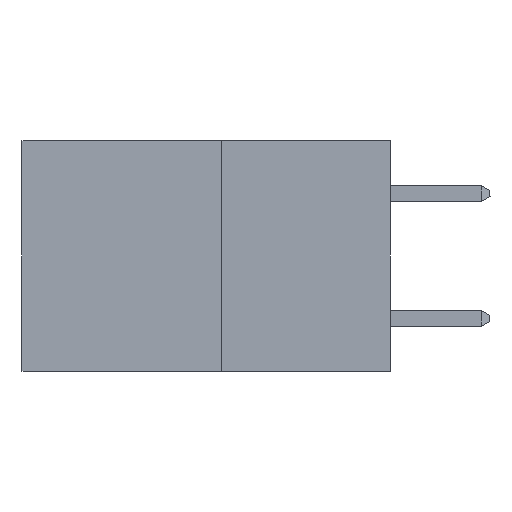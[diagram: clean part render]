
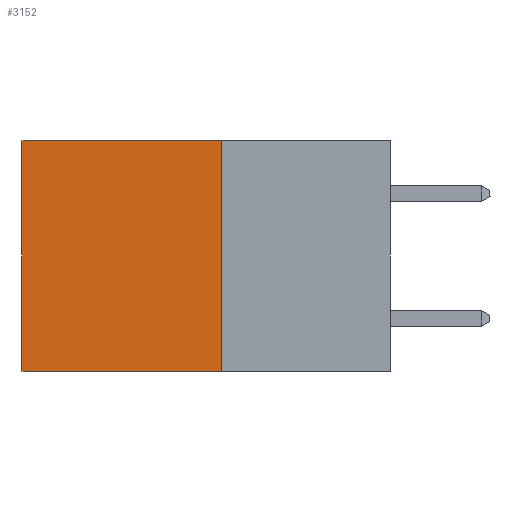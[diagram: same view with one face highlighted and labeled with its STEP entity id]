
A CAD part, left-side view. The second image highlights one B-rep face of the part: STEP entity #3152.
In plain terms, the highlighted planar face has unit normal (-1, 0, 0).
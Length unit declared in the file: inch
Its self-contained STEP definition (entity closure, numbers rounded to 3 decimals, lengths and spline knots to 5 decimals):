
#221 = LINE ( 'NONE', #6508, #7638 ) ;
#375 = DIRECTION ( 'NONE',  ( 0., 1., 0. ) ) ;
#657 = LINE ( 'NONE', #3395, #8274 ) ;
#1483 = AXIS2_PLACEMENT_3D ( 'NONE', #6103, #1688, #1674 ) ;
#1544 = LINE ( 'NONE', #1906, #3547 ) ;
#1674 = DIRECTION ( 'NONE',  ( 0., 0., -1. ) ) ;
#1688 = DIRECTION ( 'NONE',  ( 1., 0., 0. ) ) ;
#1906 = CARTESIAN_POINT ( 'NONE',  ( 0.277, 0.27, 0. ) ) ;
#1997 = ORIENTED_EDGE ( 'NONE', *, *, #3119, .F. ) ;
#2103 = VERTEX_POINT ( 'NONE', #8657 ) ;
#2217 = DIRECTION ( 'NONE',  ( 0., 1., 0. ) ) ;
#2464 = EDGE_CURVE ( 'NONE', #3460, #2103, #1544, .T. ) ;
#2699 = CARTESIAN_POINT ( 'NONE',  ( 0.277, 0.59, -0.37 ) ) ;
#3119 = EDGE_CURVE ( 'NONE', #3460, #9154, #221, .T. ) ;
#3152 = ADVANCED_FACE ( 'NONE', ( #3541 ), #9294, .F. ) ;
#3164 = LINE ( 'NONE', #4868, #7290 ) ;
#3395 = CARTESIAN_POINT ( 'NONE',  ( 0.277, 0.59, -0.37 ) ) ;
#3460 = VERTEX_POINT ( 'NONE', #7722 ) ;
#3541 = FACE_OUTER_BOUND ( 'NONE', #5500, .T. ) ;
#3547 = VECTOR ( 'NONE', #2217, 39.37008 ) ;
#3722 = ORIENTED_EDGE ( 'NONE', *, *, #4392, .T. ) ;
#4189 = ORIENTED_EDGE ( 'NONE', *, *, #2464, .T. ) ;
#4361 = EDGE_CURVE ( 'NONE', #9154, #7210, #3164, .T. ) ;
#4392 = EDGE_CURVE ( 'NONE', #2103, #7210, #657, .T. ) ;
#4868 = CARTESIAN_POINT ( 'NONE',  ( 0.277, 0.27, -0.37 ) ) ;
#5500 = EDGE_LOOP ( 'NONE', ( #3722, #9443, #1997, #4189 ) ) ;
#6103 = CARTESIAN_POINT ( 'NONE',  ( 0.277, 0.27, -0.37 ) ) ;
#6508 = CARTESIAN_POINT ( 'NONE',  ( 0.277, 0.27, -0.37 ) ) ;
#7210 = VERTEX_POINT ( 'NONE', #2699 ) ;
#7290 = VECTOR ( 'NONE', #375, 39.37008 ) ;
#7638 = VECTOR ( 'NONE', #8307, 39.37008 ) ;
#7722 = CARTESIAN_POINT ( 'NONE',  ( 0.277, 0.27, 0. ) ) ;
#8274 = VECTOR ( 'NONE', #8494, 39.37008 ) ;
#8307 = DIRECTION ( 'NONE',  ( 0., 0., -1. ) ) ;
#8494 = DIRECTION ( 'NONE',  ( 0., 0., -1. ) ) ;
#8657 = CARTESIAN_POINT ( 'NONE',  ( 0.277, 0.59, 0. ) ) ;
#9154 = VERTEX_POINT ( 'NONE', #9455 ) ;
#9294 = PLANE ( 'NONE',  #1483 ) ;
#9443 = ORIENTED_EDGE ( 'NONE', *, *, #4361, .F. ) ;
#9455 = CARTESIAN_POINT ( 'NONE',  ( 0.277, 0.27, -0.37 ) ) ;
